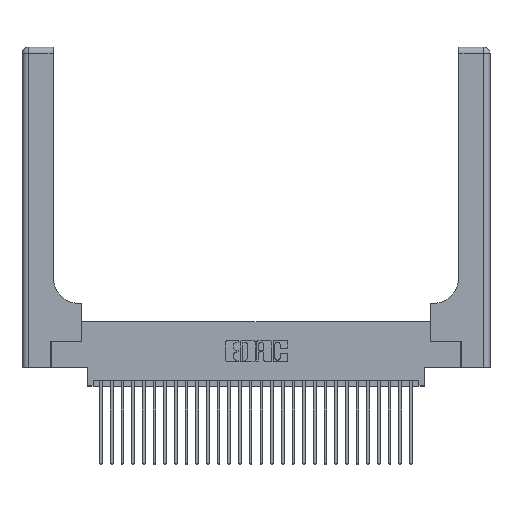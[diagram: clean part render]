
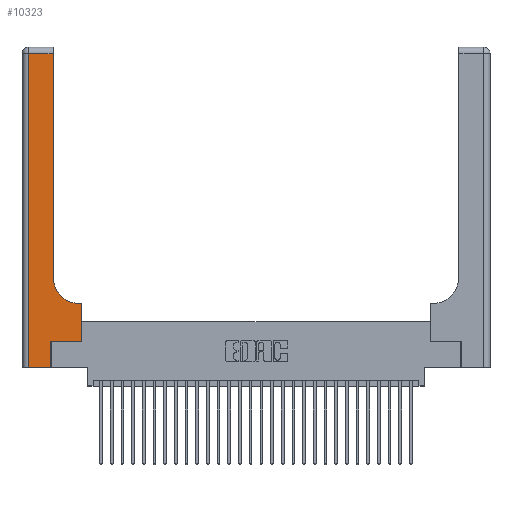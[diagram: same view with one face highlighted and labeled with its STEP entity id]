
A CAD part, top view. The second image highlights one B-rep face of the part: STEP entity #10323.
In plain terms, the highlighted planar face has unit normal (0, 0, 1).
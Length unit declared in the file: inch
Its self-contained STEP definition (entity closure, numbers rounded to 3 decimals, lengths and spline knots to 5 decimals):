
#692 = VERTEX_POINT ( 'NONE', #6264 ) ;
#739 = DIRECTION ( 'NONE',  ( -1., 0., 0. ) ) ;
#1096 = LINE ( 'NONE', #11184, #25538 ) ;
#1758 = CARTESIAN_POINT ( 'NONE',  ( 0.5585, 0.6, 0.37 ) ) ;
#2423 = DIRECTION ( 'NONE',  ( 1., 0., 0. ) ) ;
#2561 = ORIENTED_EDGE ( 'NONE', *, *, #6160, .T. ) ;
#3107 = LINE ( 'NONE', #25771, #27415 ) ;
#3400 = EDGE_CURVE ( 'NONE', #692, #18539, #11630, .T. ) ;
#3882 = CIRCLE ( 'NONE', #23999, 0.25 ) ;
#3906 = CARTESIAN_POINT ( 'NONE',  ( 0.5585, 0.25, 0.37 ) ) ;
#4099 = DIRECTION ( 'NONE',  ( 0., -1., 0. ) ) ;
#4128 = CARTESIAN_POINT ( 'NONE',  ( 0.5415, 0.6, 0.37 ) ) ;
#4847 = CARTESIAN_POINT ( 'NONE',  ( 0.269, 0., 0.37 ) ) ;
#5296 = VECTOR ( 'NONE', #7271, 39.37008 ) ;
#6160 = EDGE_CURVE ( 'NONE', #9692, #28859, #25363, .T. ) ;
#6264 = CARTESIAN_POINT ( 'NONE',  ( 0.269, 0., 0.37 ) ) ;
#7229 = VERTEX_POINT ( 'NONE', #4128 ) ;
#7271 = DIRECTION ( 'NONE',  ( 0., 1., 0. ) ) ;
#7837 = VECTOR ( 'NONE', #27111, 39.37008 ) ;
#9123 = CARTESIAN_POINT ( 'NONE',  ( 0.2915, 3., 0.37 ) ) ;
#9301 = LINE ( 'NONE', #20176, #7837 ) ;
#9379 = EDGE_CURVE ( 'NONE', #18539, #21779, #3107, .T. ) ;
#9389 = DIRECTION ( 'NONE',  ( 1., 0., 0. ) ) ;
#9692 = VERTEX_POINT ( 'NONE', #20128 ) ;
#9953 = CARTESIAN_POINT ( 'NONE',  ( 0.06, 0., 0.37 ) ) ;
#10267 = VECTOR ( 'NONE', #739, 39.37008 ) ;
#10323 = ADVANCED_FACE ( 'NONE', ( #11670 ), #26717, .F. ) ;
#10578 = EDGE_CURVE ( 'NONE', #28859, #23891, #1096, .T. ) ;
#10664 = EDGE_CURVE ( 'NONE', #14299, #9692, #24092, .T. ) ;
#11182 = ORIENTED_EDGE ( 'NONE', *, *, #9379, .T. ) ;
#11184 = CARTESIAN_POINT ( 'NONE',  ( 0.06, 3., 0.37 ) ) ;
#11630 = LINE ( 'NONE', #4847, #5296 ) ;
#11670 = FACE_OUTER_BOUND ( 'NONE', #12190, .T. ) ;
#11918 = CARTESIAN_POINT ( 'NONE',  ( 0.5415, 0.85, 0.37 ) ) ;
#12190 = EDGE_LOOP ( 'NONE', ( #15859, #2561, #17038, #23454, #24929, #11182, #28317, #18599, #14744 ) ) ;
#12772 = DIRECTION ( 'NONE',  ( 0., 0., -1. ) ) ;
#13304 = CARTESIAN_POINT ( 'NONE',  ( 0., 2.94, 0.37 ) ) ;
#14299 = VERTEX_POINT ( 'NONE', #18261 ) ;
#14319 = DIRECTION ( 'NONE',  ( 1., 0., 0. ) ) ;
#14744 = ORIENTED_EDGE ( 'NONE', *, *, #15003, .T. ) ;
#15003 = EDGE_CURVE ( 'NONE', #7229, #14299, #3882, .T. ) ;
#15259 = EDGE_CURVE ( 'NONE', #17999, #7229, #28876, .T. ) ;
#15799 = EDGE_CURVE ( 'NONE', #23891, #692, #23467, .T. ) ;
#15859 = ORIENTED_EDGE ( 'NONE', *, *, #10664, .T. ) ;
#16344 = CARTESIAN_POINT ( 'NONE',  ( 0.06, 2.94, 0.37 ) ) ;
#17038 = ORIENTED_EDGE ( 'NONE', *, *, #10578, .T. ) ;
#17738 = VECTOR ( 'NONE', #25040, 39.37008 ) ;
#17999 = VERTEX_POINT ( 'NONE', #1758 ) ;
#18261 = CARTESIAN_POINT ( 'NONE',  ( 0.2915, 0.85, 0.37 ) ) ;
#18539 = VERTEX_POINT ( 'NONE', #27043 ) ;
#18599 = ORIENTED_EDGE ( 'NONE', *, *, #15259, .T. ) ;
#19293 = EDGE_CURVE ( 'NONE', #21779, #17999, #9301, .T. ) ;
#20128 = CARTESIAN_POINT ( 'NONE',  ( 0.2915, 2.94, 0.37 ) ) ;
#20176 = CARTESIAN_POINT ( 'NONE',  ( 0.5585, 0.25, 0.37 ) ) ;
#21779 = VERTEX_POINT ( 'NONE', #3906 ) ;
#22765 = VECTOR ( 'NONE', #2423, 39.37008 ) ;
#23454 = ORIENTED_EDGE ( 'NONE', *, *, #15799, .T. ) ;
#23467 = LINE ( 'NONE', #23625, #22765 ) ;
#23625 = CARTESIAN_POINT ( 'NONE',  ( 0., 0., 0.37 ) ) ;
#23891 = VERTEX_POINT ( 'NONE', #9953 ) ;
#23999 = AXIS2_PLACEMENT_3D ( 'NONE', #11918, #28212, #14319 ) ;
#24092 = LINE ( 'NONE', #9123, #24820 ) ;
#24820 = VECTOR ( 'NONE', #25494, 39.37008 ) ;
#24929 = ORIENTED_EDGE ( 'NONE', *, *, #3400, .T. ) ;
#25040 = DIRECTION ( 'NONE',  ( -1., 0., 0. ) ) ;
#25299 = AXIS2_PLACEMENT_3D ( 'NONE', #28913, #12772, #29014 ) ;
#25363 = LINE ( 'NONE', #13304, #17738 ) ;
#25494 = DIRECTION ( 'NONE',  ( 0., 1., 0. ) ) ;
#25538 = VECTOR ( 'NONE', #4099, 39.37008 ) ;
#25771 = CARTESIAN_POINT ( 'NONE',  ( 0.269, 0.25, 0.37 ) ) ;
#26717 = PLANE ( 'NONE',  #25299 ) ;
#27043 = CARTESIAN_POINT ( 'NONE',  ( 0.269, 0.25, 0.37 ) ) ;
#27111 = DIRECTION ( 'NONE',  ( 0., 1., 0. ) ) ;
#27415 = VECTOR ( 'NONE', #9389, 39.37008 ) ;
#28212 = DIRECTION ( 'NONE',  ( 0., 0., -1. ) ) ;
#28317 = ORIENTED_EDGE ( 'NONE', *, *, #19293, .T. ) ;
#28859 = VERTEX_POINT ( 'NONE', #16344 ) ;
#28876 = LINE ( 'NONE', #28988, #10267 ) ;
#28913 = CARTESIAN_POINT ( 'NONE',  ( 0., 3., 0.37 ) ) ;
#28988 = CARTESIAN_POINT ( 'NONE',  ( 0.2915, 0.6, 0.37 ) ) ;
#29014 = DIRECTION ( 'NONE',  ( -1., 0., 0. ) ) ;
